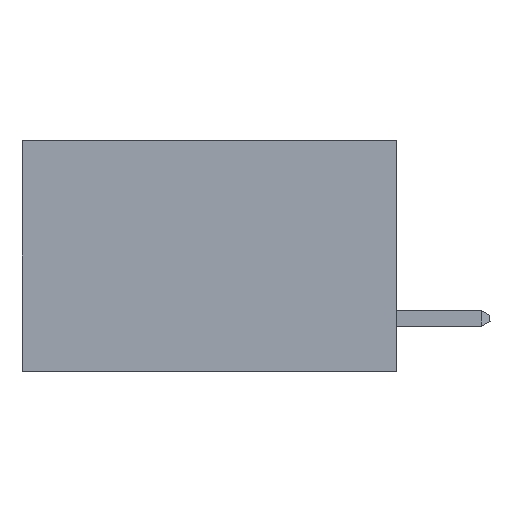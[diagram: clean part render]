
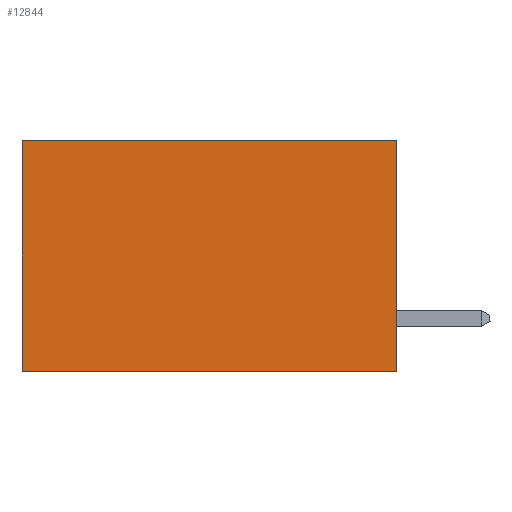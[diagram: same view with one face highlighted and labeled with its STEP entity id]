
A CAD part, left-side view. The second image highlights one B-rep face of the part: STEP entity #12844.
In plain terms, the highlighted planar face has unit normal (-1, 0, 0).
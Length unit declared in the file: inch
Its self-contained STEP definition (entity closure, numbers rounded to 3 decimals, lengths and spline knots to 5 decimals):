
#707 = EDGE_CURVE ( 'NONE', #7406, #11060, #851, .T. ) ;
#716 = VECTOR ( 'NONE', #9487, 39.37008 ) ;
#717 = CARTESIAN_POINT ( 'NONE',  ( 0.298, 0., -0.37 ) ) ;
#823 = EDGE_LOOP ( 'NONE', ( #2432, #3323, #10551, #5472 ) ) ;
#851 = LINE ( 'NONE', #6157, #11254 ) ;
#1607 = DIRECTION ( 'NONE',  ( 0., 0., -1. ) ) ;
#2407 = FACE_OUTER_BOUND ( 'NONE', #823, .T. ) ;
#2432 = ORIENTED_EDGE ( 'NONE', *, *, #9168, .T. ) ;
#3219 = LINE ( 'NONE', #5157, #5097 ) ;
#3323 = ORIENTED_EDGE ( 'NONE', *, *, #4241, .F. ) ;
#3478 = CARTESIAN_POINT ( 'NONE',  ( 0.298, 0., 0. ) ) ;
#3805 = VERTEX_POINT ( 'NONE', #4208 ) ;
#4208 = CARTESIAN_POINT ( 'NONE',  ( 0.298, 0.6, 0. ) ) ;
#4241 = EDGE_CURVE ( 'NONE', #11060, #6987, #11647, .T. ) ;
#5097 = VECTOR ( 'NONE', #12903, 39.37008 ) ;
#5157 = CARTESIAN_POINT ( 'NONE',  ( 0.298, 0.6, 0. ) ) ;
#5472 = ORIENTED_EDGE ( 'NONE', *, *, #10409, .T. ) ;
#5968 = CARTESIAN_POINT ( 'NONE',  ( 0.298, 0., 0. ) ) ;
#6157 = CARTESIAN_POINT ( 'NONE',  ( 0.298, 0., 0. ) ) ;
#6788 = LINE ( 'NONE', #5968, #11812 ) ;
#6900 = DIRECTION ( 'NONE',  ( 0., 1., 0. ) ) ;
#6987 = VERTEX_POINT ( 'NONE', #13562 ) ;
#7046 = CARTESIAN_POINT ( 'NONE',  ( 0.298, 0., -0.37 ) ) ;
#7406 = VERTEX_POINT ( 'NONE', #9756 ) ;
#7423 = AXIS2_PLACEMENT_3D ( 'NONE', #3478, #11194, #1607 ) ;
#7765 = PLANE ( 'NONE',  #7423 ) ;
#9168 = EDGE_CURVE ( 'NONE', #3805, #6987, #3219, .T. ) ;
#9487 = DIRECTION ( 'NONE',  ( 0., 1., 0. ) ) ;
#9756 = CARTESIAN_POINT ( 'NONE',  ( 0.298, 0., 0. ) ) ;
#10409 = EDGE_CURVE ( 'NONE', #7406, #3805, #6788, .T. ) ;
#10551 = ORIENTED_EDGE ( 'NONE', *, *, #707, .F. ) ;
#10623 = DIRECTION ( 'NONE',  ( 0., 0., -1. ) ) ;
#11060 = VERTEX_POINT ( 'NONE', #7046 ) ;
#11194 = DIRECTION ( 'NONE',  ( 1., 0., 0. ) ) ;
#11254 = VECTOR ( 'NONE', #10623, 39.37008 ) ;
#11647 = LINE ( 'NONE', #717, #716 ) ;
#11812 = VECTOR ( 'NONE', #6900, 39.37008 ) ;
#12844 = ADVANCED_FACE ( 'NONE', ( #2407 ), #7765, .F. ) ;
#12903 = DIRECTION ( 'NONE',  ( 0., 0., -1. ) ) ;
#13562 = CARTESIAN_POINT ( 'NONE',  ( 0.298, 0.6, -0.37 ) ) ;
